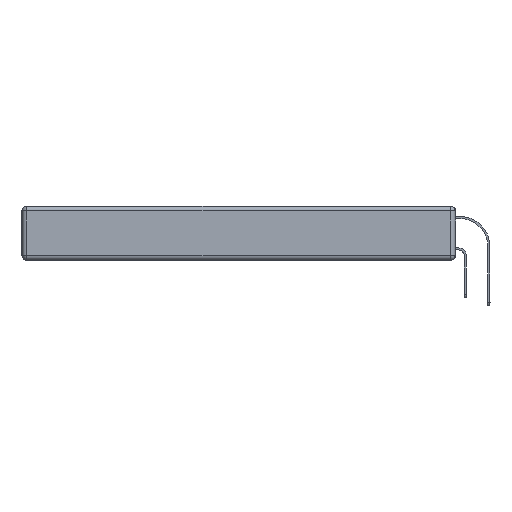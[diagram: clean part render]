
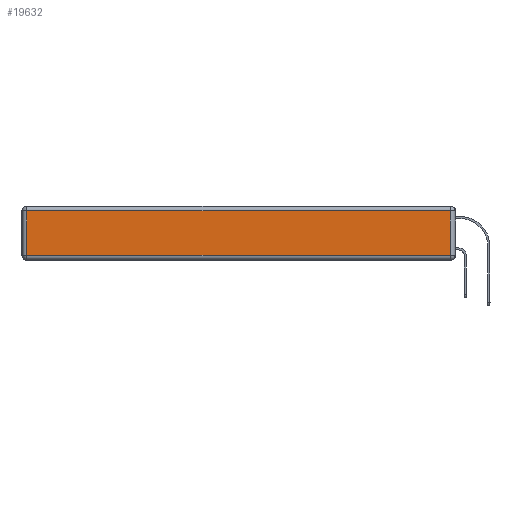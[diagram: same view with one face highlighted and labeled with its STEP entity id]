
A CAD part, left-side view. The second image highlights one B-rep face of the part: STEP entity #19632.
In plain terms, the highlighted planar face has unit normal (-1, 0, 0).
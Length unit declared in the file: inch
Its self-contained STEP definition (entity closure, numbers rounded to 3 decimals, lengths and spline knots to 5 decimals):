
#33 = CARTESIAN_POINT ( 'NONE',  ( 0., 2.72, -0.313 ) ) ;
#1230 = VECTOR ( 'NONE', #12609, 39.37008 ) ;
#1396 = VERTEX_POINT ( 'NONE', #4354 ) ;
#1874 = CARTESIAN_POINT ( 'NONE',  ( 0., 0., -0.313 ) ) ;
#3330 = LINE ( 'NONE', #22412, #1230 ) ;
#4354 = CARTESIAN_POINT ( 'NONE',  ( 0., 0.03, -0.313 ) ) ;
#4592 = EDGE_CURVE ( 'NONE', #13031, #1396, #15308, .T. ) ;
#5264 = CARTESIAN_POINT ( 'NONE',  ( 0., 2.72, -0.343 ) ) ;
#5454 = CARTESIAN_POINT ( 'NONE',  ( 0., 0., -0.343 ) ) ;
#5770 = VECTOR ( 'NONE', #20987, 39.37008 ) ;
#6785 = LINE ( 'NONE', #6926, #13623 ) ;
#6926 = CARTESIAN_POINT ( 'NONE',  ( 0., 2.75, -0.03 ) ) ;
#6930 = ORIENTED_EDGE ( 'NONE', *, *, #8744, .T. ) ;
#8744 = EDGE_CURVE ( 'NONE', #10076, #13031, #11599, .T. ) ;
#10076 = VERTEX_POINT ( 'NONE', #25043 ) ;
#10415 = VERTEX_POINT ( 'NONE', #18172 ) ;
#11375 = ORIENTED_EDGE ( 'NONE', *, *, #4592, .T. ) ;
#11599 = LINE ( 'NONE', #5264, #17450 ) ;
#12609 = DIRECTION ( 'NONE',  ( 0., 0., 1. ) ) ;
#13031 = VERTEX_POINT ( 'NONE', #33 ) ;
#13338 = DIRECTION ( 'NONE',  ( -1., 0., 0. ) ) ;
#13487 = AXIS2_PLACEMENT_3D ( 'NONE', #5454, #13338, #21191 ) ;
#13623 = VECTOR ( 'NONE', #14811, 39.37008 ) ;
#13651 = DIRECTION ( 'NONE',  ( 0., 0., -1. ) ) ;
#13661 = EDGE_CURVE ( 'NONE', #10415, #10076, #6785, .T. ) ;
#14811 = DIRECTION ( 'NONE',  ( 0., 1., 0. ) ) ;
#15269 = FACE_OUTER_BOUND ( 'NONE', #17174, .T. ) ;
#15308 = LINE ( 'NONE', #1874, #5770 ) ;
#15455 = ORIENTED_EDGE ( 'NONE', *, *, #22227, .T. ) ;
#17174 = EDGE_LOOP ( 'NONE', ( #11375, #15455, #18838, #6930 ) ) ;
#17450 = VECTOR ( 'NONE', #13651, 39.37008 ) ;
#18172 = CARTESIAN_POINT ( 'NONE',  ( 0., 0.03, -0.03 ) ) ;
#18838 = ORIENTED_EDGE ( 'NONE', *, *, #13661, .T. ) ;
#19632 = ADVANCED_FACE ( 'NONE', ( #15269 ), #23139, .T. ) ;
#20987 = DIRECTION ( 'NONE',  ( 0., -1., 0. ) ) ;
#21191 = DIRECTION ( 'NONE',  ( 0., 0., 1. ) ) ;
#22227 = EDGE_CURVE ( 'NONE', #1396, #10415, #3330, .T. ) ;
#22412 = CARTESIAN_POINT ( 'NONE',  ( 0., 0.03, -0.343 ) ) ;
#23139 = PLANE ( 'NONE',  #13487 ) ;
#25043 = CARTESIAN_POINT ( 'NONE',  ( 0., 2.72, -0.03 ) ) ;
